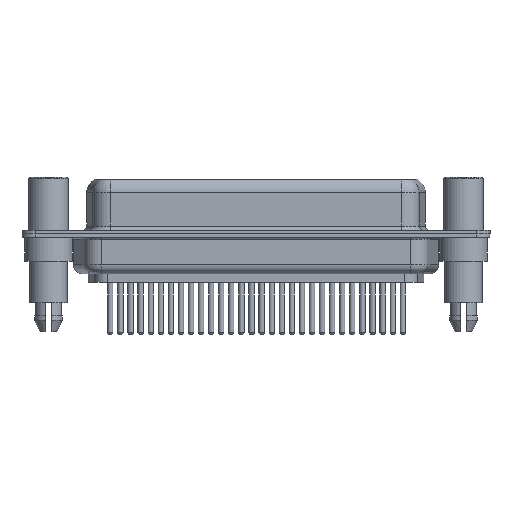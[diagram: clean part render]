
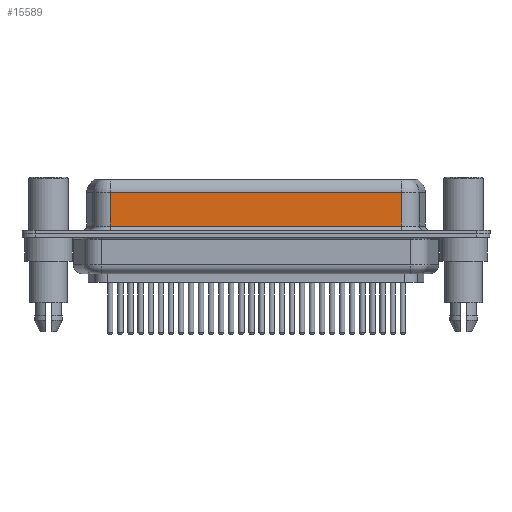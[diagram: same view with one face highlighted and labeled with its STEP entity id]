
A CAD part, front view. The second image highlights one B-rep face of the part: STEP entity #15589.
In plain terms, the highlighted planar face has unit normal (0, -1, 0).
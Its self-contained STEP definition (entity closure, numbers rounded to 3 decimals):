
#44 = VECTOR ( 'NONE', #13959, 1000. ) ;
#363 = ORIENTED_EDGE ( 'NONE', *, *, #25148, .T. ) ;
#645 = ORIENTED_EDGE ( 'NONE', *, *, #2329, .F. ) ;
#1541 = VERTEX_POINT ( 'NONE', #12913 ) ;
#2105 = EDGE_CURVE ( 'NONE', #30718, #3298, #25615, .T. ) ;
#2329 = EDGE_CURVE ( 'NONE', #30718, #1541, #24325, .T. ) ;
#2403 = DIRECTION ( 'NONE',  ( 0., 0., 1. ) ) ;
#2697 = CARTESIAN_POINT ( 'NONE',  ( 7.013, -3.95, 0.9 ) ) ;
#3298 = VERTEX_POINT ( 'NONE', #26078 ) ;
#3687 = LINE ( 'NONE', #8154, #13021 ) ;
#5118 = PLANE ( 'NONE',  #11870 ) ;
#7488 = DIRECTION ( 'NONE',  ( 0., 1., 0. ) ) ;
#7720 = LINE ( 'NONE', #17481, #9463 ) ;
#8154 = CARTESIAN_POINT ( 'NONE',  ( 7.013, -3.95, 6.4 ) ) ;
#8189 = CARTESIAN_POINT ( 'NONE',  ( 40.037, -3.95, 6.4 ) ) ;
#9463 = VECTOR ( 'NONE', #24818, 1000. ) ;
#10256 = VERTEX_POINT ( 'NONE', #2697 ) ;
#11184 = DIRECTION ( 'NONE',  ( 0., 0., -1. ) ) ;
#11870 = AXIS2_PLACEMENT_3D ( 'NONE', #21727, #7488, #2403 ) ;
#12838 = DIRECTION ( 'NONE',  ( 0., 0., -1. ) ) ;
#12913 = CARTESIAN_POINT ( 'NONE',  ( 40.037, -3.95, 0.9 ) ) ;
#13021 = VECTOR ( 'NONE', #11184, 1000. ) ;
#13959 = DIRECTION ( 'NONE',  ( -1., 0., 0. ) ) ;
#15589 = ADVANCED_FACE ( 'NONE', ( #16934 ), #5118, .F. ) ;
#16934 = FACE_OUTER_BOUND ( 'NONE', #29616, .T. ) ;
#17481 = CARTESIAN_POINT ( 'NONE',  ( 40.037, -3.95, 0.9 ) ) ;
#18504 = ORIENTED_EDGE ( 'NONE', *, *, #2105, .T. ) ;
#18689 = CARTESIAN_POINT ( 'NONE',  ( 40.037, -3.95, 4.65 ) ) ;
#21000 = CARTESIAN_POINT ( 'NONE',  ( 40.037, -3.95, 4.65 ) ) ;
#21727 = CARTESIAN_POINT ( 'NONE',  ( 40.037, -3.95, 6.4 ) ) ;
#24325 = LINE ( 'NONE', #8189, #30387 ) ;
#24818 = DIRECTION ( 'NONE',  ( 1., 0., 0. ) ) ;
#25148 = EDGE_CURVE ( 'NONE', #3298, #10256, #3687, .T. ) ;
#25615 = LINE ( 'NONE', #21000, #44 ) ;
#25896 = EDGE_CURVE ( 'NONE', #10256, #1541, #7720, .T. ) ;
#26078 = CARTESIAN_POINT ( 'NONE',  ( 7.013, -3.95, 4.65 ) ) ;
#26777 = ORIENTED_EDGE ( 'NONE', *, *, #25896, .T. ) ;
#29616 = EDGE_LOOP ( 'NONE', ( #645, #18504, #363, #26777 ) ) ;
#30387 = VECTOR ( 'NONE', #12838, 1000. ) ;
#30718 = VERTEX_POINT ( 'NONE', #18689 ) ;
